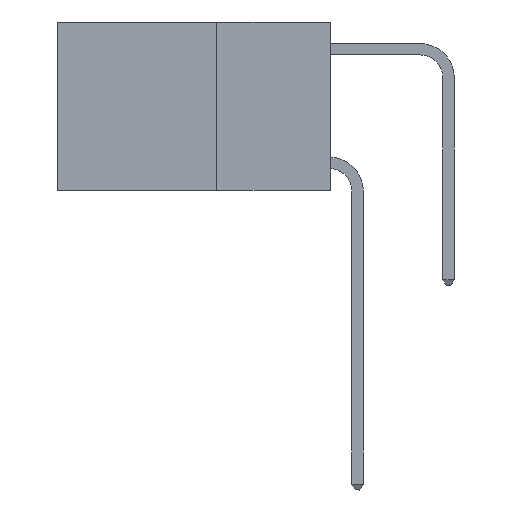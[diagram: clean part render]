
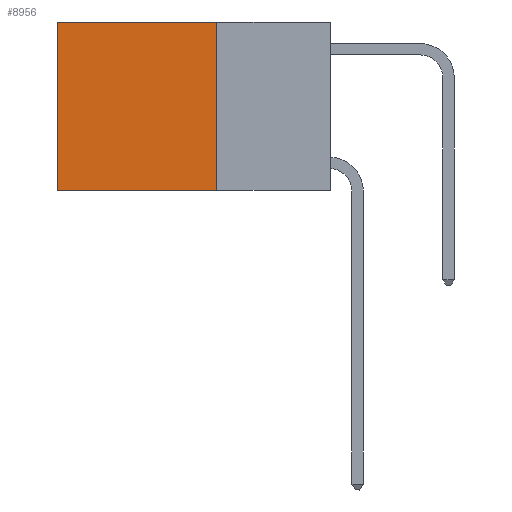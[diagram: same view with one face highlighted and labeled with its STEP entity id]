
A CAD part, left-side view. The second image highlights one B-rep face of the part: STEP entity #8956.
In plain terms, the highlighted planar face has unit normal (-1, 0, 0).
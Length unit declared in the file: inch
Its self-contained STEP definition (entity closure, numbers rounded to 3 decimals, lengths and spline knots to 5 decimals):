
#603 = VERTEX_POINT ( 'NONE', #6148 ) ;
#720 = VECTOR ( 'NONE', #15547, 39.37008 ) ;
#1659 = ORIENTED_EDGE ( 'NONE', *, *, #17022, .F. ) ;
#2453 = ORIENTED_EDGE ( 'NONE', *, *, #9684, .T. ) ;
#3270 = DIRECTION ( 'NONE',  ( 1., 0., 0. ) ) ;
#3767 = VECTOR ( 'NONE', #5185, 39.37008 ) ;
#5185 = DIRECTION ( 'NONE',  ( 0., 1., 0. ) ) ;
#5186 = DIRECTION ( 'NONE',  ( 0., 0., -1. ) ) ;
#6054 = LINE ( 'NONE', #19460, #720 ) ;
#6063 = ORIENTED_EDGE ( 'NONE', *, *, #25321, .T. ) ;
#6148 = CARTESIAN_POINT ( 'NONE',  ( 0.2625, 0.6, -0.37 ) ) ;
#6771 = ORIENTED_EDGE ( 'NONE', *, *, #18623, .F. ) ;
#7142 = CARTESIAN_POINT ( 'NONE',  ( 0.2625, 0.25, 0. ) ) ;
#8956 = ADVANCED_FACE ( 'NONE', ( #20646 ), #25066, .F. ) ;
#9684 = EDGE_CURVE ( 'NONE', #15063, #15201, #19068, .T. ) ;
#11149 = DIRECTION ( 'NONE',  ( 0., 0., -1. ) ) ;
#11785 = VECTOR ( 'NONE', #5186, 39.37008 ) ;
#12190 = VECTOR ( 'NONE', #11149, 39.37008 ) ;
#13568 = CARTESIAN_POINT ( 'NONE',  ( 0.2625, 0.25, 0. ) ) ;
#15063 = VERTEX_POINT ( 'NONE', #13568 ) ;
#15201 = VERTEX_POINT ( 'NONE', #17654 ) ;
#15229 = CARTESIAN_POINT ( 'NONE',  ( 0.2625, 0.25, 0. ) ) ;
#15365 = AXIS2_PLACEMENT_3D ( 'NONE', #15229, #3270, #17231 ) ;
#15547 = DIRECTION ( 'NONE',  ( 0., 1., 0. ) ) ;
#17022 = EDGE_CURVE ( 'NONE', #15063, #20026, #17064, .T. ) ;
#17064 = LINE ( 'NONE', #7142, #11785 ) ;
#17133 = CARTESIAN_POINT ( 'NONE',  ( 0.2625, 0.25, 0. ) ) ;
#17231 = DIRECTION ( 'NONE',  ( 0., 0., -1. ) ) ;
#17654 = CARTESIAN_POINT ( 'NONE',  ( 0.2625, 0.6, 0. ) ) ;
#18106 = LINE ( 'NONE', #20987, #12190 ) ;
#18623 = EDGE_CURVE ( 'NONE', #20026, #603, #6054, .T. ) ;
#19068 = LINE ( 'NONE', #17133, #3767 ) ;
#19460 = CARTESIAN_POINT ( 'NONE',  ( 0.2625, 0.25, -0.37 ) ) ;
#20026 = VERTEX_POINT ( 'NONE', #23593 ) ;
#20646 = FACE_OUTER_BOUND ( 'NONE', #23830, .T. ) ;
#20987 = CARTESIAN_POINT ( 'NONE',  ( 0.2625, 0.6, 0. ) ) ;
#23593 = CARTESIAN_POINT ( 'NONE',  ( 0.2625, 0.25, -0.37 ) ) ;
#23830 = EDGE_LOOP ( 'NONE', ( #6063, #6771, #1659, #2453 ) ) ;
#25066 = PLANE ( 'NONE',  #15365 ) ;
#25321 = EDGE_CURVE ( 'NONE', #15201, #603, #18106, .T. ) ;
